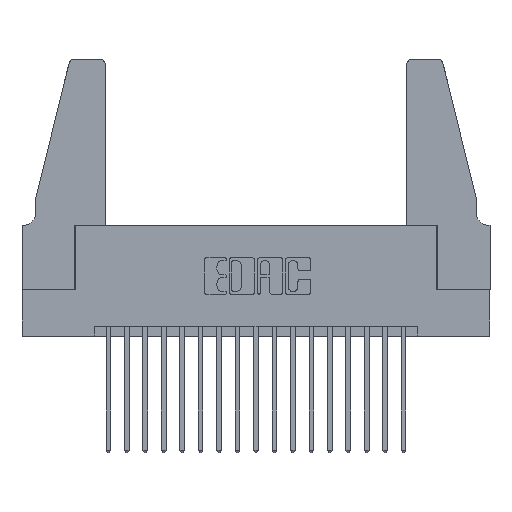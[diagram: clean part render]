
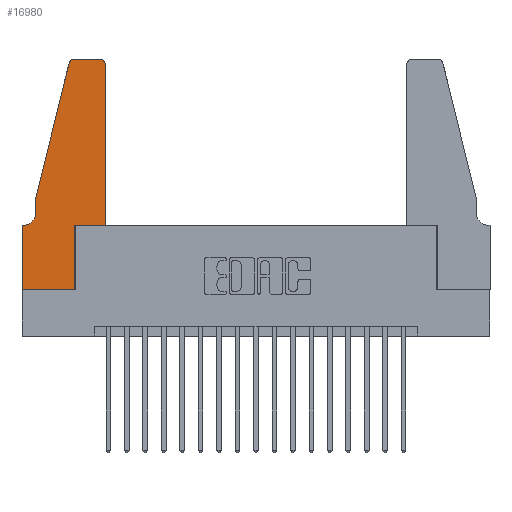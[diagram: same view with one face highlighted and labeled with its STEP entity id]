
A CAD part, top view. The second image highlights one B-rep face of the part: STEP entity #16980.
In plain terms, the highlighted planar face has unit normal (0, 0, 1).
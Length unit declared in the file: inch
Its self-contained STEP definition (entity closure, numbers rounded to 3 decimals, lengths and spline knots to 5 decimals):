
#23 = ORIENTED_EDGE ( 'NONE', *, *, #18378, .T. ) ;
#247 = AXIS2_PLACEMENT_3D ( 'NONE', #981, #2598, #12723 ) ;
#621 = VERTEX_POINT ( 'NONE', #13956 ) ;
#981 = CARTESIAN_POINT ( 'NONE',  ( 0., 0.35, 0.37 ) ) ;
#1017 = ORIENTED_EDGE ( 'NONE', *, *, #10996, .T. ) ;
#1287 = EDGE_CURVE ( 'NONE', #16103, #9179, #10030, .T. ) ;
#1496 = LINE ( 'NONE', #11841, #16465 ) ;
#1505 = DIRECTION ( 'NONE',  ( 0., 0., 1. ) ) ;
#1591 = LINE ( 'NONE', #6703, #12748 ) ;
#1614 = VERTEX_POINT ( 'NONE', #9121 ) ;
#1620 = DIRECTION ( 'NONE',  ( -0.239, -0.971, 0. ) ) ;
#1641 = VERTEX_POINT ( 'NONE', #18028 ) ;
#1748 = CARTESIAN_POINT ( 'NONE',  ( 0.284, 1.25, 0.37 ) ) ;
#2039 = CARTESIAN_POINT ( 'NONE',  ( 0.0755, 0.42, 0.37 ) ) ;
#2598 = DIRECTION ( 'NONE',  ( 0., 0., 1. ) ) ;
#3302 = DIRECTION ( 'NONE',  ( 0., 1., 0. ) ) ;
#3755 = CARTESIAN_POINT ( 'NONE',  ( 0.4505, 0.35, 0.37 ) ) ;
#4282 = EDGE_CURVE ( 'NONE', #621, #1641, #10375, .T. ) ;
#4462 = CARTESIAN_POINT ( 'NONE',  ( 0.0755, 0.35, 0.37 ) ) ;
#4876 = VECTOR ( 'NONE', #3302, 39.37008 ) ;
#5077 = CARTESIAN_POINT ( 'NONE',  ( 0., 0., 0.37 ) ) ;
#5274 = CARTESIAN_POINT ( 'NONE',  ( 0.2865, 0., 0.37 ) ) ;
#5431 = EDGE_CURVE ( 'NONE', #17940, #7272, #14310, .T. ) ;
#5541 = EDGE_LOOP ( 'NONE', ( #17149, #7143, #18514, #11348, #23, #12226, #1017, #9770, #13999, #10676, #14445, #14885 ) ) ;
#5577 = DIRECTION ( 'NONE',  ( -1., 0., 0. ) ) ;
#5711 = EDGE_CURVE ( 'NONE', #10063, #13243, #1591, .T. ) ;
#5833 = CARTESIAN_POINT ( 'NONE',  ( 0.4505, 0.35, 0.37 ) ) ;
#6126 = CARTESIAN_POINT ( 'NONE',  ( 0.0055, 0.42, 0.37 ) ) ;
#6593 = DIRECTION ( 'NONE',  ( 0., 0., 1. ) ) ;
#6703 = CARTESIAN_POINT ( 'NONE',  ( 0.0755, 0.5, 0.37 ) ) ;
#7143 = ORIENTED_EDGE ( 'NONE', *, *, #5431, .T. ) ;
#7272 = VERTEX_POINT ( 'NONE', #11560 ) ;
#7289 = EDGE_CURVE ( 'NONE', #1614, #11700, #16730, .T. ) ;
#7541 = DIRECTION ( 'NONE',  ( -1., 0., 0. ) ) ;
#7821 = AXIS2_PLACEMENT_3D ( 'NONE', #6126, #16062, #7541 ) ;
#8044 = EDGE_CURVE ( 'NONE', #1641, #17940, #15112, .T. ) ;
#8259 = LINE ( 'NONE', #11967, #4876 ) ;
#8550 = CARTESIAN_POINT ( 'NONE',  ( 0., 0.35, 0.37 ) ) ;
#8916 = LINE ( 'NONE', #3755, #12242 ) ;
#9121 = CARTESIAN_POINT ( 'NONE',  ( 0.0055, 0.35, 0.37 ) ) ;
#9179 = VERTEX_POINT ( 'NONE', #5274 ) ;
#9770 = ORIENTED_EDGE ( 'NONE', *, *, #1287, .T. ) ;
#10030 = LINE ( 'NONE', #5077, #17189 ) ;
#10049 = DIRECTION ( 'NONE',  ( 0., 1., 0. ) ) ;
#10063 = VERTEX_POINT ( 'NONE', #18625 ) ;
#10309 = CARTESIAN_POINT ( 'NONE',  ( 0.284, 1.22, 0.37 ) ) ;
#10375 = CIRCLE ( 'NONE', #15224, 0.03 ) ;
#10676 = ORIENTED_EDGE ( 'NONE', *, *, #16180, .T. ) ;
#10996 = EDGE_CURVE ( 'NONE', #11700, #16103, #12859, .T. ) ;
#11137 = EDGE_CURVE ( 'NONE', #11243, #621, #18251, .T. ) ;
#11243 = VERTEX_POINT ( 'NONE', #18880 ) ;
#11348 = ORIENTED_EDGE ( 'NONE', *, *, #5711, .T. ) ;
#11560 = CARTESIAN_POINT ( 'NONE',  ( 0.25487, 1.22718, 0.37 ) ) ;
#11629 = VERTEX_POINT ( 'NONE', #18360 ) ;
#11700 = VERTEX_POINT ( 'NONE', #8550 ) ;
#11736 = DIRECTION ( 'NONE',  ( 1., 0., 0. ) ) ;
#11841 = CARTESIAN_POINT ( 'NONE',  ( 0.0755, 0.5, 0.37 ) ) ;
#11967 = CARTESIAN_POINT ( 'NONE',  ( 0.2865, 0.35, 0.37 ) ) ;
#12226 = ORIENTED_EDGE ( 'NONE', *, *, #7289, .T. ) ;
#12242 = VECTOR ( 'NONE', #13793, 39.37008 ) ;
#12407 = VECTOR ( 'NONE', #12662, 39.37008 ) ;
#12481 = FACE_OUTER_BOUND ( 'NONE', #5541, .T. ) ;
#12599 = CARTESIAN_POINT ( 'NONE',  ( 0., 0., 0.37 ) ) ;
#12658 = CARTESIAN_POINT ( 'NONE',  ( 0.2605, 1.25, 0.37 ) ) ;
#12662 = DIRECTION ( 'NONE',  ( 0., -1., 0. ) ) ;
#12723 = DIRECTION ( 'NONE',  ( 1., 0., 0. ) ) ;
#12748 = VECTOR ( 'NONE', #18110, 39.37008 ) ;
#12859 = LINE ( 'NONE', #12599, #12407 ) ;
#13243 = VERTEX_POINT ( 'NONE', #2039 ) ;
#13343 = CIRCLE ( 'NONE', #7821, 0.07 ) ;
#13793 = DIRECTION ( 'NONE',  ( 1., 0., 0. ) ) ;
#13953 = VECTOR ( 'NONE', #10049, 39.37008 ) ;
#13956 = CARTESIAN_POINT ( 'NONE',  ( 0.4505, 1.22, 0.37 ) ) ;
#13999 = ORIENTED_EDGE ( 'NONE', *, *, #15953, .T. ) ;
#14310 = CIRCLE ( 'NONE', #17044, 0.03 ) ;
#14445 = ORIENTED_EDGE ( 'NONE', *, *, #11137, .T. ) ;
#14885 = ORIENTED_EDGE ( 'NONE', *, *, #4282, .T. ) ;
#15053 = CARTESIAN_POINT ( 'NONE',  ( 0., 0., 0.37 ) ) ;
#15088 = CARTESIAN_POINT ( 'NONE',  ( 0.4205, 1.22, 0.37 ) ) ;
#15112 = LINE ( 'NONE', #12658, #18504 ) ;
#15224 = AXIS2_PLACEMENT_3D ( 'NONE', #15088, #6593, #16538 ) ;
#15903 = DIRECTION ( 'NONE',  ( -1., 0., 0. ) ) ;
#15905 = EDGE_CURVE ( 'NONE', #7272, #10063, #1496, .T. ) ;
#15953 = EDGE_CURVE ( 'NONE', #9179, #11629, #8259, .T. ) ;
#16062 = DIRECTION ( 'NONE',  ( 0., 0., -1. ) ) ;
#16103 = VERTEX_POINT ( 'NONE', #15053 ) ;
#16180 = EDGE_CURVE ( 'NONE', #11629, #11243, #8916, .T. ) ;
#16263 = VECTOR ( 'NONE', #15903, 39.37008 ) ;
#16465 = VECTOR ( 'NONE', #1620, 39.37008 ) ;
#16538 = DIRECTION ( 'NONE',  ( 1., 0., 0. ) ) ;
#16730 = LINE ( 'NONE', #4462, #16263 ) ;
#16959 = DIRECTION ( 'NONE',  ( 1., 0., 0. ) ) ;
#16980 = ADVANCED_FACE ( 'NONE', ( #12481 ), #18445, .T. ) ;
#17044 = AXIS2_PLACEMENT_3D ( 'NONE', #10309, #1505, #11736 ) ;
#17149 = ORIENTED_EDGE ( 'NONE', *, *, #8044, .T. ) ;
#17189 = VECTOR ( 'NONE', #16959, 39.37008 ) ;
#17940 = VERTEX_POINT ( 'NONE', #1748 ) ;
#18028 = CARTESIAN_POINT ( 'NONE',  ( 0.4205, 1.25, 0.37 ) ) ;
#18110 = DIRECTION ( 'NONE',  ( 0., -1., 0. ) ) ;
#18251 = LINE ( 'NONE', #5833, #13953 ) ;
#18360 = CARTESIAN_POINT ( 'NONE',  ( 0.2865, 0.35, 0.37 ) ) ;
#18378 = EDGE_CURVE ( 'NONE', #13243, #1614, #13343, .T. ) ;
#18445 = PLANE ( 'NONE',  #247 ) ;
#18504 = VECTOR ( 'NONE', #5577, 39.37008 ) ;
#18514 = ORIENTED_EDGE ( 'NONE', *, *, #15905, .T. ) ;
#18625 = CARTESIAN_POINT ( 'NONE',  ( 0.0755, 0.5, 0.37 ) ) ;
#18880 = CARTESIAN_POINT ( 'NONE',  ( 0.4505, 0.35, 0.37 ) ) ;
